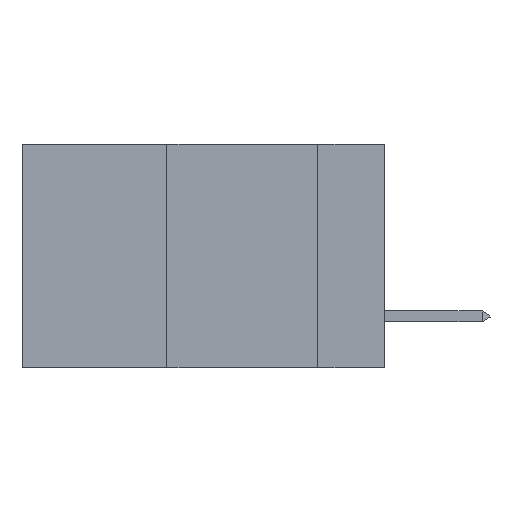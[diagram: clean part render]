
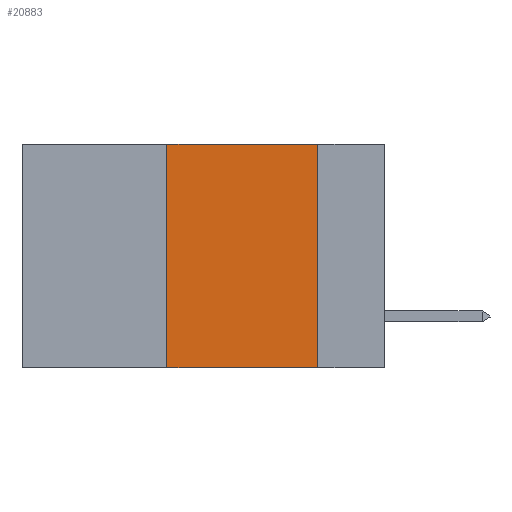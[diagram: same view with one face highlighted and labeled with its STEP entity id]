
A CAD part, left-side view. The second image highlights one B-rep face of the part: STEP entity #20883.
In plain terms, the highlighted planar face has unit normal (-1, 0, 0).
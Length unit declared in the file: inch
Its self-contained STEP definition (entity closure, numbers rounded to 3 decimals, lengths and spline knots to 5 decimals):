
#1951 = VERTEX_POINT ( 'NONE', #7177 ) ;
#2272 = EDGE_CURVE ( 'NONE', #19708, #1951, #14450, .T. ) ;
#3221 = EDGE_CURVE ( 'NONE', #31031, #1951, #21720, .T. ) ;
#3924 = CARTESIAN_POINT ( 'NONE',  ( 0., 0.36, 0. ) ) ;
#4137 = CARTESIAN_POINT ( 'NONE',  ( 0., 0.36, 0. ) ) ;
#4365 = DIRECTION ( 'NONE',  ( 0., 0., 1. ) ) ;
#5330 = CARTESIAN_POINT ( 'NONE',  ( 0., 0.11, 0. ) ) ;
#5526 = ORIENTED_EDGE ( 'NONE', *, *, #17730, .F. ) ;
#7034 = CARTESIAN_POINT ( 'NONE',  ( 0., 0.6, 0. ) ) ;
#7177 = CARTESIAN_POINT ( 'NONE',  ( 0., 0.11, -0.37 ) ) ;
#7656 = VECTOR ( 'NONE', #25754, 39.37008 ) ;
#8157 = ORIENTED_EDGE ( 'NONE', *, *, #3221, .T. ) ;
#8924 = EDGE_CURVE ( 'NONE', #31031, #22016, #23863, .T. ) ;
#9114 = AXIS2_PLACEMENT_3D ( 'NONE', #7034, #22330, #22218 ) ;
#9247 = CARTESIAN_POINT ( 'NONE',  ( 0., 0.36, -0.37 ) ) ;
#11285 = VECTOR ( 'NONE', #20904, 39.37008 ) ;
#11730 = CARTESIAN_POINT ( 'NONE',  ( 0., 0.6, -0.37 ) ) ;
#12995 = ORIENTED_EDGE ( 'NONE', *, *, #2272, .F. ) ;
#13572 = FACE_OUTER_BOUND ( 'NONE', #29048, .T. ) ;
#14450 = LINE ( 'NONE', #5330, #7656 ) ;
#15265 = LINE ( 'NONE', #25852, #11285 ) ;
#17182 = CARTESIAN_POINT ( 'NONE',  ( 0., 0.11, 0. ) ) ;
#17730 = EDGE_CURVE ( 'NONE', #22016, #19708, #15265, .T. ) ;
#19708 = VERTEX_POINT ( 'NONE', #17182 ) ;
#20883 = ADVANCED_FACE ( 'NONE', ( #13572 ), #27705, .F. ) ;
#20904 = DIRECTION ( 'NONE',  ( 0., -1., 0. ) ) ;
#21720 = LINE ( 'NONE', #11730, #27360 ) ;
#22016 = VERTEX_POINT ( 'NONE', #3924 ) ;
#22218 = DIRECTION ( 'NONE',  ( 0., 0., -1. ) ) ;
#22330 = DIRECTION ( 'NONE',  ( 1., 0., 0. ) ) ;
#23863 = LINE ( 'NONE', #4137, #31444 ) ;
#24614 = ORIENTED_EDGE ( 'NONE', *, *, #8924, .F. ) ;
#25754 = DIRECTION ( 'NONE',  ( 0., 0., -1. ) ) ;
#25852 = CARTESIAN_POINT ( 'NONE',  ( 0., 0.6, 0. ) ) ;
#26597 = DIRECTION ( 'NONE',  ( 0., -1., 0. ) ) ;
#27360 = VECTOR ( 'NONE', #26597, 39.37008 ) ;
#27705 = PLANE ( 'NONE',  #9114 ) ;
#29048 = EDGE_LOOP ( 'NONE', ( #12995, #5526, #24614, #8157 ) ) ;
#31031 = VERTEX_POINT ( 'NONE', #9247 ) ;
#31444 = VECTOR ( 'NONE', #4365, 39.37008 ) ;
